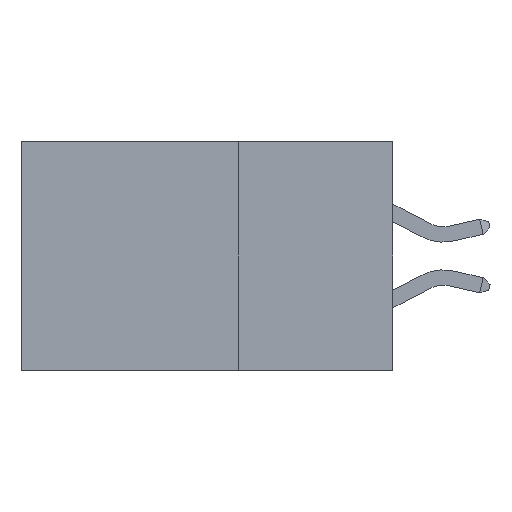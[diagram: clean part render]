
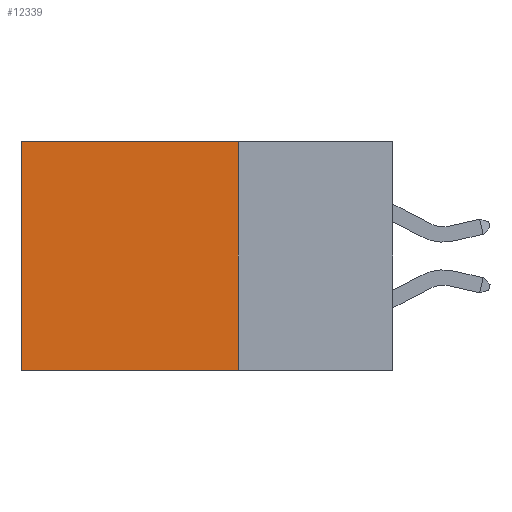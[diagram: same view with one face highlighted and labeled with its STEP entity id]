
A CAD part, left-side view. The second image highlights one B-rep face of the part: STEP entity #12339.
In plain terms, the highlighted planar face has unit normal (-1, 0, 0).
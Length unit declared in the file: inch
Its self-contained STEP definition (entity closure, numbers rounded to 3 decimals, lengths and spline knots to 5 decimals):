
#1295 = CARTESIAN_POINT ( 'NONE',  ( 0.2875, 0.25, 0. ) ) ;
#1729 = CARTESIAN_POINT ( 'NONE',  ( 0.2875, 0.25, 0. ) ) ;
#2424 = AXIS2_PLACEMENT_3D ( 'NONE', #17158, #15503, #5040 ) ;
#2516 = ORIENTED_EDGE ( 'NONE', *, *, #3844, .T. ) ;
#3587 = DIRECTION ( 'NONE',  ( 0., 1., 0. ) ) ;
#3844 = EDGE_CURVE ( 'NONE', #8469, #16291, #7700, .T. ) ;
#5040 = DIRECTION ( 'NONE',  ( 0., 0., -1. ) ) ;
#5414 = EDGE_CURVE ( 'NONE', #18944, #16291, #8170, .T. ) ;
#5629 = LINE ( 'NONE', #1729, #14378 ) ;
#6146 = EDGE_CURVE ( 'NONE', #9707, #8469, #5629, .T. ) ;
#7052 = CARTESIAN_POINT ( 'NONE',  ( 0.2875, 0.25, 0. ) ) ;
#7690 = ORIENTED_EDGE ( 'NONE', *, *, #14377, .F. ) ;
#7700 = LINE ( 'NONE', #18336, #16403 ) ;
#8170 = LINE ( 'NONE', #12173, #20793 ) ;
#8469 = VERTEX_POINT ( 'NONE', #10053 ) ;
#8547 = ORIENTED_EDGE ( 'NONE', *, *, #5414, .F. ) ;
#9707 = VERTEX_POINT ( 'NONE', #1295 ) ;
#10053 = CARTESIAN_POINT ( 'NONE',  ( 0.2875, 0.6, 0. ) ) ;
#12173 = CARTESIAN_POINT ( 'NONE',  ( 0.2875, 0.25, -0.37 ) ) ;
#12339 = ADVANCED_FACE ( 'NONE', ( #16210 ), #13790, .F. ) ;
#13790 = PLANE ( 'NONE',  #2424 ) ;
#13979 = LINE ( 'NONE', #7052, #22418 ) ;
#14377 = EDGE_CURVE ( 'NONE', #9707, #18944, #13979, .T. ) ;
#14378 = VECTOR ( 'NONE', #3587, 39.37008 ) ;
#15205 = CARTESIAN_POINT ( 'NONE',  ( 0.2875, 0.25, -0.37 ) ) ;
#15503 = DIRECTION ( 'NONE',  ( 1., 0., 0. ) ) ;
#15550 = ORIENTED_EDGE ( 'NONE', *, *, #6146, .T. ) ;
#15742 = EDGE_LOOP ( 'NONE', ( #2516, #8547, #7690, #15550 ) ) ;
#16210 = FACE_OUTER_BOUND ( 'NONE', #15742, .T. ) ;
#16291 = VERTEX_POINT ( 'NONE', #21882 ) ;
#16403 = VECTOR ( 'NONE', #21704, 39.37008 ) ;
#17158 = CARTESIAN_POINT ( 'NONE',  ( 0.2875, 0.25, 0. ) ) ;
#18336 = CARTESIAN_POINT ( 'NONE',  ( 0.2875, 0.6, 0. ) ) ;
#18944 = VERTEX_POINT ( 'NONE', #15205 ) ;
#20793 = VECTOR ( 'NONE', #22348, 39.37008 ) ;
#21704 = DIRECTION ( 'NONE',  ( 0., 0., -1. ) ) ;
#21882 = CARTESIAN_POINT ( 'NONE',  ( 0.2875, 0.6, -0.37 ) ) ;
#22348 = DIRECTION ( 'NONE',  ( 0., 1., 0. ) ) ;
#22418 = VECTOR ( 'NONE', #22488, 39.37008 ) ;
#22488 = DIRECTION ( 'NONE',  ( 0., 0., -1. ) ) ;
